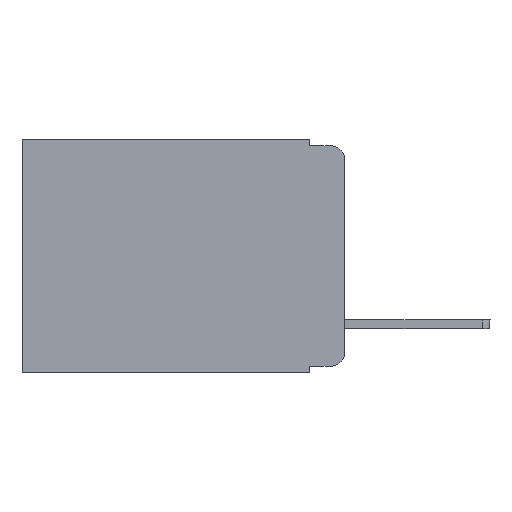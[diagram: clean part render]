
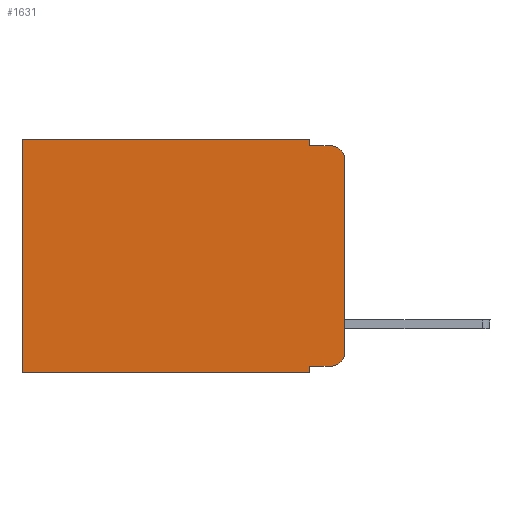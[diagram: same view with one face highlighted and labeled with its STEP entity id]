
A CAD part, left-side view. The second image highlights one B-rep face of the part: STEP entity #1631.
In plain terms, the highlighted planar face has unit normal (-1, 0, 0).
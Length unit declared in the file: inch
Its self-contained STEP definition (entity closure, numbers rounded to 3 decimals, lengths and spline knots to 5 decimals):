
#309 = EDGE_CURVE ( 'NONE', #15257, #5833, #17141, .T. ) ;
#321 = VERTEX_POINT ( 'NONE', #2591 ) ;
#412 = ORIENTED_EDGE ( 'NONE', *, *, #1544, .F. ) ;
#1544 = EDGE_CURVE ( 'NONE', #4159, #15557, #12367, .T. ) ;
#1631 = ADVANCED_FACE ( 'NONE', ( #2189 ), #7534, .F. ) ;
#1936 = DIRECTION ( 'NONE',  ( 0., -1., 0. ) ) ;
#1970 = CIRCLE ( 'NONE', #11764, 0.02 ) ;
#2189 = FACE_OUTER_BOUND ( 'NONE', #9106, .T. ) ;
#2374 = CARTESIAN_POINT ( 'NONE',  ( 0.298, 0.473, 0. ) ) ;
#2591 = CARTESIAN_POINT ( 'NONE',  ( 0.298, 0., -0.313 ) ) ;
#2802 = DIRECTION ( 'NONE',  ( 0., 0., -1. ) ) ;
#2830 = VECTOR ( 'NONE', #16557, 39.37008 ) ;
#2855 = VECTOR ( 'NONE', #7322, 39.37008 ) ;
#2892 = CARTESIAN_POINT ( 'NONE',  ( 0.298, 0., 0. ) ) ;
#3433 = DIRECTION ( 'NONE',  ( 0., 0., -1. ) ) ;
#3518 = CARTESIAN_POINT ( 'NONE',  ( 0.298, 0.02, -0.313 ) ) ;
#3826 = VERTEX_POINT ( 'NONE', #2374 ) ;
#3926 = EDGE_CURVE ( 'NONE', #4427, #321, #6926, .T. ) ;
#3960 = ORIENTED_EDGE ( 'NONE', *, *, #13011, .T. ) ;
#4109 = ORIENTED_EDGE ( 'NONE', *, *, #8121, .F. ) ;
#4159 = VERTEX_POINT ( 'NONE', #11824 ) ;
#4427 = VERTEX_POINT ( 'NONE', #4704 ) ;
#4604 = LINE ( 'NONE', #15568, #2855 ) ;
#4704 = CARTESIAN_POINT ( 'NONE',  ( 0.298, 0., -0.03 ) ) ;
#4707 = ORIENTED_EDGE ( 'NONE', *, *, #7611, .T. ) ;
#4857 = VECTOR ( 'NONE', #13950, 39.37008 ) ;
#5106 = LINE ( 'NONE', #7740, #6829 ) ;
#5250 = LINE ( 'NONE', #14385, #14972 ) ;
#5833 = VERTEX_POINT ( 'NONE', #9514 ) ;
#6041 = CIRCLE ( 'NONE', #13888, 0.02 ) ;
#6043 = DIRECTION ( 'NONE',  ( 0., 1., 0. ) ) ;
#6131 = EDGE_CURVE ( 'NONE', #8649, #7607, #5106, .T. ) ;
#6472 = VECTOR ( 'NONE', #6043, 39.37008 ) ;
#6829 = VECTOR ( 'NONE', #7998, 39.37008 ) ;
#6926 = LINE ( 'NONE', #2892, #16304 ) ;
#7020 = CARTESIAN_POINT ( 'NONE',  ( 0.298, 0.051, -0.01 ) ) ;
#7322 = DIRECTION ( 'NONE',  ( 0., 1., 0. ) ) ;
#7534 = PLANE ( 'NONE',  #8226 ) ;
#7607 = VERTEX_POINT ( 'NONE', #11423 ) ;
#7611 = EDGE_CURVE ( 'NONE', #7607, #321, #6041, .T. ) ;
#7740 = CARTESIAN_POINT ( 'NONE',  ( 0.298, 0.051, -0.333 ) ) ;
#7998 = DIRECTION ( 'NONE',  ( 0., -1., 0. ) ) ;
#8121 = EDGE_CURVE ( 'NONE', #8649, #15257, #5250, .T. ) ;
#8226 = AXIS2_PLACEMENT_3D ( 'NONE', #14467, #14293, #12876 ) ;
#8500 = VERTEX_POINT ( 'NONE', #8985 ) ;
#8649 = VERTEX_POINT ( 'NONE', #10731 ) ;
#8759 = CARTESIAN_POINT ( 'NONE',  ( 0.298, 0., -0.343 ) ) ;
#8814 = ORIENTED_EDGE ( 'NONE', *, *, #309, .F. ) ;
#8960 = DIRECTION ( 'NONE',  ( -1., 0., 0. ) ) ;
#8985 = CARTESIAN_POINT ( 'NONE',  ( 0.298, 0.02, -0.01 ) ) ;
#9106 = EDGE_LOOP ( 'NONE', ( #14336, #3960, #15173, #412, #9808, #15228, #8814, #4109, #16857, #4707 ) ) ;
#9514 = CARTESIAN_POINT ( 'NONE',  ( 0.298, 0.473, -0.343 ) ) ;
#9791 = EDGE_CURVE ( 'NONE', #4159, #3826, #4604, .T. ) ;
#9808 = ORIENTED_EDGE ( 'NONE', *, *, #9791, .T. ) ;
#9816 = CARTESIAN_POINT ( 'NONE',  ( 0.298, 0.051, 0. ) ) ;
#10731 = CARTESIAN_POINT ( 'NONE',  ( 0.298, 0.051, -0.333 ) ) ;
#11423 = CARTESIAN_POINT ( 'NONE',  ( 0.298, 0.02, -0.333 ) ) ;
#11764 = AXIS2_PLACEMENT_3D ( 'NONE', #11770, #17112, #12114 ) ;
#11770 = CARTESIAN_POINT ( 'NONE',  ( 0.298, 0.02, -0.03 ) ) ;
#11824 = CARTESIAN_POINT ( 'NONE',  ( 0.298, 0.051, 0. ) ) ;
#12114 = DIRECTION ( 'NONE',  ( 0., 0., -1. ) ) ;
#12367 = LINE ( 'NONE', #9816, #4857 ) ;
#12451 = LINE ( 'NONE', #12607, #2830 ) ;
#12607 = CARTESIAN_POINT ( 'NONE',  ( 0.298, 0.473, 0. ) ) ;
#12876 = DIRECTION ( 'NONE',  ( 0., 0., -1. ) ) ;
#13011 = EDGE_CURVE ( 'NONE', #4427, #8500, #1970, .T. ) ;
#13478 = CARTESIAN_POINT ( 'NONE',  ( 0.298, 0.051, -0.01 ) ) ;
#13888 = AXIS2_PLACEMENT_3D ( 'NONE', #3518, #8960, #3433 ) ;
#13950 = DIRECTION ( 'NONE',  ( 0., 0., -1. ) ) ;
#14293 = DIRECTION ( 'NONE',  ( 1., 0., 0. ) ) ;
#14336 = ORIENTED_EDGE ( 'NONE', *, *, #3926, .F. ) ;
#14385 = CARTESIAN_POINT ( 'NONE',  ( 0.298, 0.051, 0. ) ) ;
#14467 = CARTESIAN_POINT ( 'NONE',  ( 0.298, 0., 0. ) ) ;
#14551 = DIRECTION ( 'NONE',  ( 0., 0., -1. ) ) ;
#14734 = EDGE_CURVE ( 'NONE', #15557, #8500, #15099, .T. ) ;
#14972 = VECTOR ( 'NONE', #14551, 39.37008 ) ;
#15099 = LINE ( 'NONE', #7020, #15986 ) ;
#15173 = ORIENTED_EDGE ( 'NONE', *, *, #14734, .F. ) ;
#15177 = EDGE_CURVE ( 'NONE', #3826, #5833, #12451, .T. ) ;
#15228 = ORIENTED_EDGE ( 'NONE', *, *, #15177, .T. ) ;
#15251 = CARTESIAN_POINT ( 'NONE',  ( 0.298, 0.051, -0.343 ) ) ;
#15257 = VERTEX_POINT ( 'NONE', #15251 ) ;
#15557 = VERTEX_POINT ( 'NONE', #13478 ) ;
#15568 = CARTESIAN_POINT ( 'NONE',  ( 0.298, 0., 0. ) ) ;
#15986 = VECTOR ( 'NONE', #1936, 39.37008 ) ;
#16304 = VECTOR ( 'NONE', #2802, 39.37008 ) ;
#16557 = DIRECTION ( 'NONE',  ( 0., 0., -1. ) ) ;
#16857 = ORIENTED_EDGE ( 'NONE', *, *, #6131, .T. ) ;
#17112 = DIRECTION ( 'NONE',  ( -1., 0., 0. ) ) ;
#17141 = LINE ( 'NONE', #8759, #6472 ) ;
